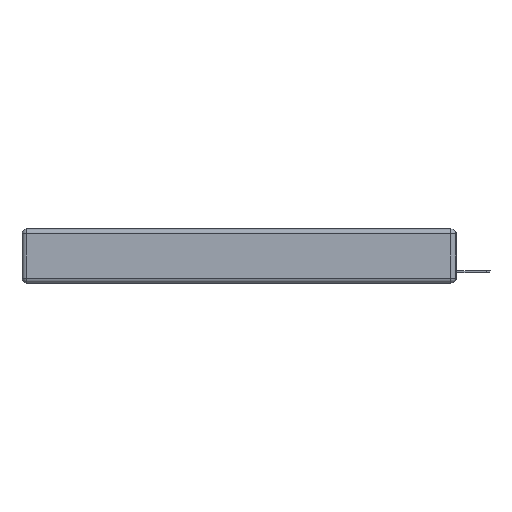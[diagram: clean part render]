
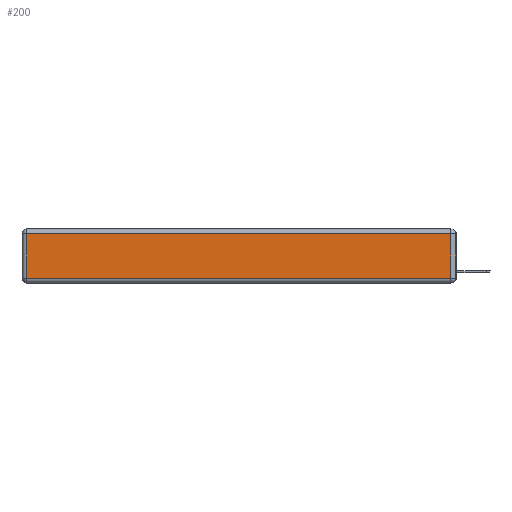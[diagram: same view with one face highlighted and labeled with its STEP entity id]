
A CAD part, left-side view. The second image highlights one B-rep face of the part: STEP entity #200.
In plain terms, the highlighted planar face has unit normal (-1, 0, 0).
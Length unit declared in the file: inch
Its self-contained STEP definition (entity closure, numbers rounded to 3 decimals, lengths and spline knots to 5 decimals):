
#48 = DIRECTION ( 'NONE',  ( -1., 0., 0. ) ) ;
#200 = ADVANCED_FACE ( 'NONE', ( #8904 ), #9570, .T. ) ;
#786 = ORIENTED_EDGE ( 'NONE', *, *, #11831, .T. ) ;
#921 = EDGE_CURVE ( 'NONE', #8067, #3243, #1173, .T. ) ;
#962 = VECTOR ( 'NONE', #11738, 39.37008 ) ;
#1173 = LINE ( 'NONE', #1312, #2656 ) ;
#1312 = CARTESIAN_POINT ( 'NONE',  ( 0., 0., -0.313 ) ) ;
#1372 = VECTOR ( 'NONE', #2696, 39.37008 ) ;
#1555 = VERTEX_POINT ( 'NONE', #1716 ) ;
#1716 = CARTESIAN_POINT ( 'NONE',  ( 0., 0.03, -0.03 ) ) ;
#1905 = CARTESIAN_POINT ( 'NONE',  ( 0., 0., -0.343 ) ) ;
#1945 = LINE ( 'NONE', #4429, #1372 ) ;
#2318 = CARTESIAN_POINT ( 'NONE',  ( 0., 2.75, -0.03 ) ) ;
#2656 = VECTOR ( 'NONE', #4124, 39.37008 ) ;
#2696 = DIRECTION ( 'NONE',  ( 0., 0., -1. ) ) ;
#2920 = CARTESIAN_POINT ( 'NONE',  ( 0., 0.03, -0.313 ) ) ;
#2976 = CARTESIAN_POINT ( 'NONE',  ( 0., 0.03, -0.343 ) ) ;
#3243 = VERTEX_POINT ( 'NONE', #2920 ) ;
#3633 = VECTOR ( 'NONE', #8832, 39.37008 ) ;
#4124 = DIRECTION ( 'NONE',  ( 0., -1., 0. ) ) ;
#4256 = AXIS2_PLACEMENT_3D ( 'NONE', #1905, #48, #4755 ) ;
#4429 = CARTESIAN_POINT ( 'NONE',  ( 0., 2.72, -0.343 ) ) ;
#4755 = DIRECTION ( 'NONE',  ( 0., 0., 1. ) ) ;
#7505 = CARTESIAN_POINT ( 'NONE',  ( 0., 2.72, -0.313 ) ) ;
#8067 = VERTEX_POINT ( 'NONE', #7505 ) ;
#8389 = LINE ( 'NONE', #2318, #962 ) ;
#8697 = ORIENTED_EDGE ( 'NONE', *, *, #8879, .T. ) ;
#8832 = DIRECTION ( 'NONE',  ( 0., 0., 1. ) ) ;
#8879 = EDGE_CURVE ( 'NONE', #3243, #1555, #8983, .T. ) ;
#8904 = FACE_OUTER_BOUND ( 'NONE', #11260, .T. ) ;
#8983 = LINE ( 'NONE', #2976, #3633 ) ;
#9570 = PLANE ( 'NONE',  #4256 ) ;
#9993 = CARTESIAN_POINT ( 'NONE',  ( 0., 2.72, -0.03 ) ) ;
#10003 = ORIENTED_EDGE ( 'NONE', *, *, #921, .T. ) ;
#10414 = ORIENTED_EDGE ( 'NONE', *, *, #12108, .T. ) ;
#10504 = VERTEX_POINT ( 'NONE', #9993 ) ;
#11260 = EDGE_LOOP ( 'NONE', ( #10003, #8697, #786, #10414 ) ) ;
#11738 = DIRECTION ( 'NONE',  ( 0., 1., 0. ) ) ;
#11831 = EDGE_CURVE ( 'NONE', #1555, #10504, #8389, .T. ) ;
#12108 = EDGE_CURVE ( 'NONE', #10504, #8067, #1945, .T. ) ;
